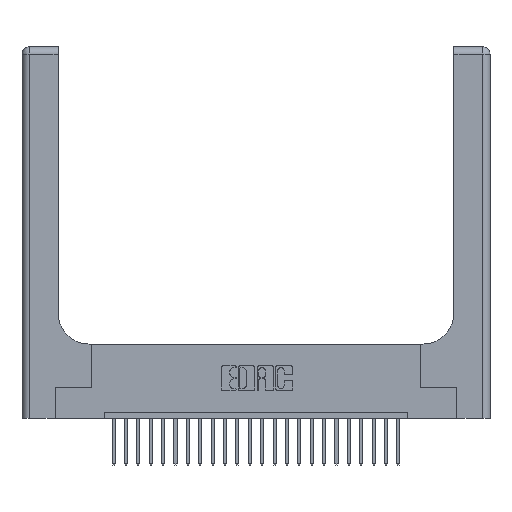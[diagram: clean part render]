
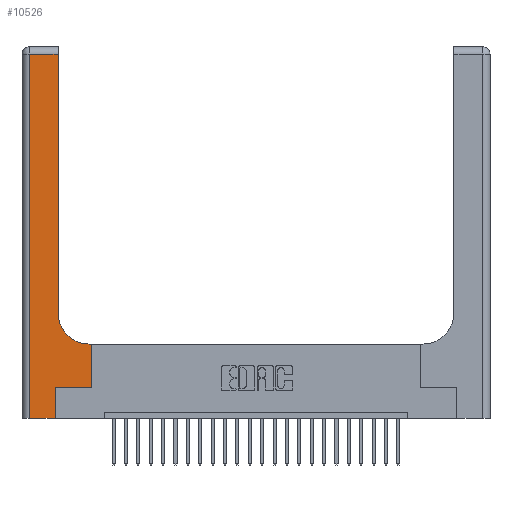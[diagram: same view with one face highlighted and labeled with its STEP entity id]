
A CAD part, top view. The second image highlights one B-rep face of the part: STEP entity #10526.
In plain terms, the highlighted planar face has unit normal (0, 0, 1).
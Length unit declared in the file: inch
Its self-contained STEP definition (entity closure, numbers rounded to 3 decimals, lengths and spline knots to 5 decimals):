
#19 = DIRECTION ( 'NONE',  ( -1., 0., 0. ) ) ;
#397 = LINE ( 'NONE', #12379, #23372 ) ;
#413 = CARTESIAN_POINT ( 'NONE',  ( 0.5585, 0.25, 0.37 ) ) ;
#591 = DIRECTION ( 'NONE',  ( 0., 1., 0. ) ) ;
#612 = CARTESIAN_POINT ( 'NONE',  ( 0.2915, 2.94, 0.37 ) ) ;
#629 = VECTOR ( 'NONE', #591, 39.37008 ) ;
#857 = EDGE_CURVE ( 'NONE', #16957, #9449, #397, .T. ) ;
#936 = VECTOR ( 'NONE', #15393, 39.37008 ) ;
#1234 = ORIENTED_EDGE ( 'NONE', *, *, #11230, .T. ) ;
#1561 = EDGE_CURVE ( 'NONE', #9449, #9306, #24885, .T. ) ;
#1685 = CARTESIAN_POINT ( 'NONE',  ( 0.5585, 0.6, 0.37 ) ) ;
#2435 = VECTOR ( 'NONE', #10021, 39.37008 ) ;
#2566 = VERTEX_POINT ( 'NONE', #1685 ) ;
#2663 = CARTESIAN_POINT ( 'NONE',  ( 0., 2.94, 0.37 ) ) ;
#3015 = CARTESIAN_POINT ( 'NONE',  ( 0.5415, 0.85, 0.37 ) ) ;
#4641 = ORIENTED_EDGE ( 'NONE', *, *, #19548, .T. ) ;
#5245 = VERTEX_POINT ( 'NONE', #13750 ) ;
#6137 = DIRECTION ( 'NONE',  ( 0., 0., -1. ) ) ;
#6302 = VERTEX_POINT ( 'NONE', #612 ) ;
#6455 = DIRECTION ( 'NONE',  ( 0., -1., 0. ) ) ;
#6658 = DIRECTION ( 'NONE',  ( 1., 0., 0. ) ) ;
#7131 = VECTOR ( 'NONE', #7796, 39.37008 ) ;
#7363 = VERTEX_POINT ( 'NONE', #25712 ) ;
#7759 = LINE ( 'NONE', #11640, #7131 ) ;
#7796 = DIRECTION ( 'NONE',  ( 0., 1., 0. ) ) ;
#7919 = AXIS2_PLACEMENT_3D ( 'NONE', #3015, #8724, #6658 ) ;
#8724 = DIRECTION ( 'NONE',  ( 0., 0., -1. ) ) ;
#9306 = VERTEX_POINT ( 'NONE', #22081 ) ;
#9341 = VECTOR ( 'NONE', #16457, 39.37008 ) ;
#9449 = VERTEX_POINT ( 'NONE', #23199 ) ;
#9552 = ORIENTED_EDGE ( 'NONE', *, *, #857, .T. ) ;
#9905 = CARTESIAN_POINT ( 'NONE',  ( 0., 0., 0.37 ) ) ;
#10021 = DIRECTION ( 'NONE',  ( -1., 0., 0. ) ) ;
#10059 = CARTESIAN_POINT ( 'NONE',  ( 0.2915, 0.85, 0.37 ) ) ;
#10109 = CARTESIAN_POINT ( 'NONE',  ( 0.2915, 0.6, 0.37 ) ) ;
#10304 = ORIENTED_EDGE ( 'NONE', *, *, #20453, .T. ) ;
#10358 = CARTESIAN_POINT ( 'NONE',  ( 0.5585, 0.25, 0.37 ) ) ;
#10526 = ADVANCED_FACE ( 'NONE', ( #23582 ), #11890, .F. ) ;
#10584 = ORIENTED_EDGE ( 'NONE', *, *, #16510, .T. ) ;
#10627 = DIRECTION ( 'NONE',  ( 1., 0., 0. ) ) ;
#10716 = EDGE_CURVE ( 'NONE', #5245, #23002, #18583, .T. ) ;
#11131 = LINE ( 'NONE', #10109, #2435 ) ;
#11230 = EDGE_CURVE ( 'NONE', #2566, #5245, #11131, .T. ) ;
#11640 = CARTESIAN_POINT ( 'NONE',  ( 0.269, 0., 0.37 ) ) ;
#11890 = PLANE ( 'NONE',  #17736 ) ;
#12379 = CARTESIAN_POINT ( 'NONE',  ( 0.06, 3., 0.37 ) ) ;
#13383 = CARTESIAN_POINT ( 'NONE',  ( 0.2915, 3., 0.37 ) ) ;
#13385 = LINE ( 'NONE', #18679, #21163 ) ;
#13750 = CARTESIAN_POINT ( 'NONE',  ( 0.5415, 0.6, 0.37 ) ) ;
#13804 = DIRECTION ( 'NONE',  ( 1., 0., 0. ) ) ;
#14115 = VERTEX_POINT ( 'NONE', #10358 ) ;
#14451 = EDGE_LOOP ( 'NONE', ( #24365, #4641, #9552, #16451, #10584, #18752, #10304, #1234, #16422 ) ) ;
#15393 = DIRECTION ( 'NONE',  ( 0., 1., 0. ) ) ;
#15864 = EDGE_CURVE ( 'NONE', #7363, #14115, #13385, .T. ) ;
#16422 = ORIENTED_EDGE ( 'NONE', *, *, #10716, .T. ) ;
#16451 = ORIENTED_EDGE ( 'NONE', *, *, #1561, .T. ) ;
#16457 = DIRECTION ( 'NONE',  ( -1., 0., 0. ) ) ;
#16510 = EDGE_CURVE ( 'NONE', #9306, #7363, #7759, .T. ) ;
#16957 = VERTEX_POINT ( 'NONE', #24964 ) ;
#17736 = AXIS2_PLACEMENT_3D ( 'NONE', #20021, #6137, #19 ) ;
#18360 = VECTOR ( 'NONE', #13804, 39.37008 ) ;
#18583 = CIRCLE ( 'NONE', #7919, 0.25 ) ;
#18679 = CARTESIAN_POINT ( 'NONE',  ( 0.269, 0.25, 0.37 ) ) ;
#18752 = ORIENTED_EDGE ( 'NONE', *, *, #15864, .T. ) ;
#19218 = LINE ( 'NONE', #13383, #936 ) ;
#19548 = EDGE_CURVE ( 'NONE', #6302, #16957, #25217, .T. ) ;
#20021 = CARTESIAN_POINT ( 'NONE',  ( 0., 3., 0.37 ) ) ;
#20453 = EDGE_CURVE ( 'NONE', #14115, #2566, #21737, .T. ) ;
#20741 = EDGE_CURVE ( 'NONE', #23002, #6302, #19218, .T. ) ;
#21163 = VECTOR ( 'NONE', #10627, 39.37008 ) ;
#21737 = LINE ( 'NONE', #413, #629 ) ;
#22081 = CARTESIAN_POINT ( 'NONE',  ( 0.269, 0., 0.37 ) ) ;
#23002 = VERTEX_POINT ( 'NONE', #10059 ) ;
#23199 = CARTESIAN_POINT ( 'NONE',  ( 0.06, 0., 0.37 ) ) ;
#23372 = VECTOR ( 'NONE', #6455, 39.37008 ) ;
#23582 = FACE_OUTER_BOUND ( 'NONE', #14451, .T. ) ;
#24365 = ORIENTED_EDGE ( 'NONE', *, *, #20741, .T. ) ;
#24885 = LINE ( 'NONE', #9905, #18360 ) ;
#24964 = CARTESIAN_POINT ( 'NONE',  ( 0.06, 2.94, 0.37 ) ) ;
#25217 = LINE ( 'NONE', #2663, #9341 ) ;
#25712 = CARTESIAN_POINT ( 'NONE',  ( 0.269, 0.25, 0.37 ) ) ;
